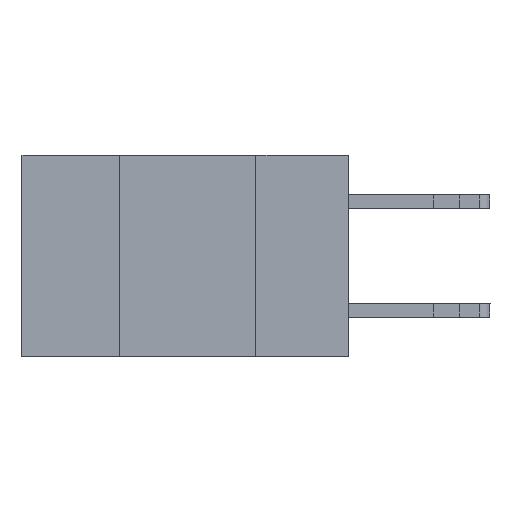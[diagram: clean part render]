
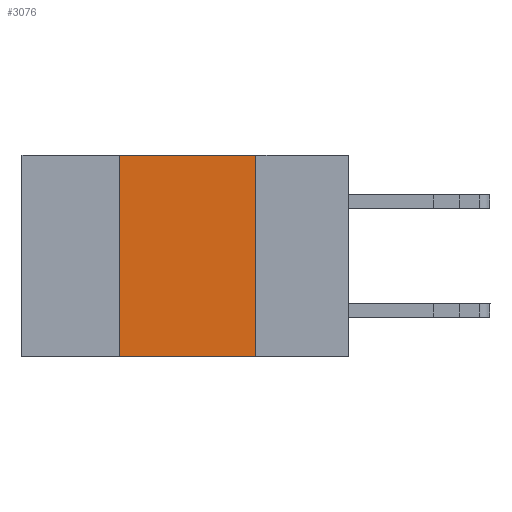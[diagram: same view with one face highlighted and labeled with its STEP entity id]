
A CAD part, left-side view. The second image highlights one B-rep face of the part: STEP entity #3076.
In plain terms, the highlighted planar face has unit normal (-1, 0, 0).
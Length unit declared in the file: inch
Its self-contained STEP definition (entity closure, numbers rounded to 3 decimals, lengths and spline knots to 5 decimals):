
#111 = CARTESIAN_POINT ( 'NONE',  ( 0., 0.17, 0. ) ) ;
#1131 = VECTOR ( 'NONE', #7337, 39.37008 ) ;
#2695 = LINE ( 'NONE', #111, #1131 ) ;
#3008 = CARTESIAN_POINT ( 'NONE',  ( 0., 0.6, 0. ) ) ;
#3076 = ADVANCED_FACE ( 'NONE', ( #8078 ), #15303, .F. ) ;
#3576 = ORIENTED_EDGE ( 'NONE', *, *, #8852, .F. ) ;
#4423 = LINE ( 'NONE', #14754, #6530 ) ;
#5518 = CARTESIAN_POINT ( 'NONE',  ( 0., 0.42, 0. ) ) ;
#6530 = VECTOR ( 'NONE', #7294, 39.37008 ) ;
#6712 = CARTESIAN_POINT ( 'NONE',  ( 0., 0.42, 0. ) ) ;
#7294 = DIRECTION ( 'NONE',  ( 0., -1., 0. ) ) ;
#7337 = DIRECTION ( 'NONE',  ( 0., 0., -1. ) ) ;
#7417 = ORIENTED_EDGE ( 'NONE', *, *, #12808, .T. ) ;
#7499 = DIRECTION ( 'NONE',  ( 0., -1., 0. ) ) ;
#8078 = FACE_OUTER_BOUND ( 'NONE', #8216, .T. ) ;
#8216 = EDGE_LOOP ( 'NONE', ( #3576, #8828, #17685, #7417 ) ) ;
#8273 = EDGE_CURVE ( 'NONE', #16067, #16864, #9706, .T. ) ;
#8307 = VECTOR ( 'NONE', #18263, 39.37008 ) ;
#8828 = ORIENTED_EDGE ( 'NONE', *, *, #15529, .F. ) ;
#8852 = EDGE_CURVE ( 'NONE', #16849, #10919, #2695, .T. ) ;
#9367 = VECTOR ( 'NONE', #7499, 39.37008 ) ;
#9706 = LINE ( 'NONE', #6712, #8307 ) ;
#10919 = VERTEX_POINT ( 'NONE', #15550 ) ;
#12808 = EDGE_CURVE ( 'NONE', #16067, #10919, #4423, .T. ) ;
#13658 = CARTESIAN_POINT ( 'NONE',  ( 0., 0.6, 0. ) ) ;
#14754 = CARTESIAN_POINT ( 'NONE',  ( 0., 0.6, -0.37 ) ) ;
#15303 = PLANE ( 'NONE',  #17098 ) ;
#15366 = DIRECTION ( 'NONE',  ( 1., 0., 0. ) ) ;
#15529 = EDGE_CURVE ( 'NONE', #16864, #16849, #15965, .T. ) ;
#15550 = CARTESIAN_POINT ( 'NONE',  ( 0., 0.17, -0.37 ) ) ;
#15965 = LINE ( 'NONE', #3008, #9367 ) ;
#16012 = CARTESIAN_POINT ( 'NONE',  ( 0., 0.17, 0. ) ) ;
#16067 = VERTEX_POINT ( 'NONE', #17112 ) ;
#16782 = DIRECTION ( 'NONE',  ( 0., 0., -1. ) ) ;
#16849 = VERTEX_POINT ( 'NONE', #16012 ) ;
#16864 = VERTEX_POINT ( 'NONE', #5518 ) ;
#17098 = AXIS2_PLACEMENT_3D ( 'NONE', #13658, #15366, #16782 ) ;
#17112 = CARTESIAN_POINT ( 'NONE',  ( 0., 0.42, -0.37 ) ) ;
#17685 = ORIENTED_EDGE ( 'NONE', *, *, #8273, .F. ) ;
#18263 = DIRECTION ( 'NONE',  ( 0., 0., 1. ) ) ;
